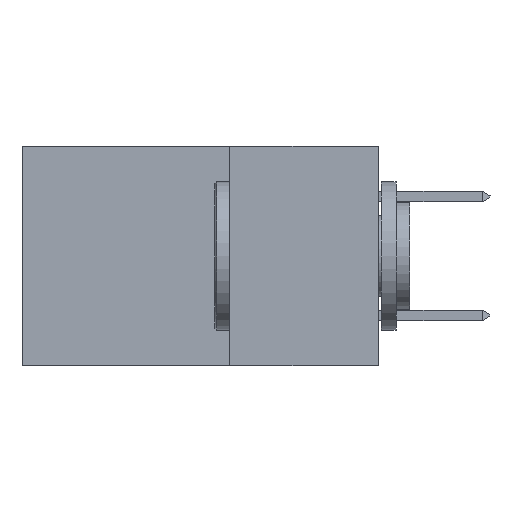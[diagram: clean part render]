
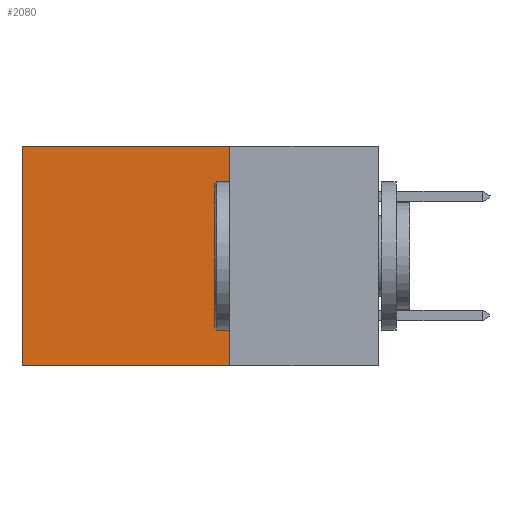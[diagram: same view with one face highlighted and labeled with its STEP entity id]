
A CAD part, left-side view. The second image highlights one B-rep face of the part: STEP entity #2080.
In plain terms, the highlighted planar face has unit normal (-1, 0, 0).
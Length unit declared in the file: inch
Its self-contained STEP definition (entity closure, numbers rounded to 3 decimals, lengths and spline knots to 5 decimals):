
#318 = DIRECTION ( 'NONE',  ( 1., 0., 0. ) ) ;
#596 = EDGE_CURVE ( 'NONE', #10384, #10099, #8486, .T. ) ;
#719 = CARTESIAN_POINT ( 'NONE',  ( 0.2615, 0.25, 0. ) ) ;
#1499 = CARTESIAN_POINT ( 'NONE',  ( 0.2615, 0.25, 0. ) ) ;
#1875 = CARTESIAN_POINT ( 'NONE',  ( 0.2615, 0.25, -0.37 ) ) ;
#2080 = ADVANCED_FACE ( 'NONE', ( #8927 ), #8737, .F. ) ;
#2107 = EDGE_LOOP ( 'NONE', ( #5415, #2706, #9807, #5911 ) ) ;
#2665 = VECTOR ( 'NONE', #9935, 39.37008 ) ;
#2706 = ORIENTED_EDGE ( 'NONE', *, *, #596, .F. ) ;
#3731 = CARTESIAN_POINT ( 'NONE',  ( 0.2615, 0.25, -0.37 ) ) ;
#4138 = AXIS2_PLACEMENT_3D ( 'NONE', #11734, #318, #5097 ) ;
#4532 = CARTESIAN_POINT ( 'NONE',  ( 0.2615, 0.6, -0.37 ) ) ;
#4996 = VERTEX_POINT ( 'NONE', #10766 ) ;
#5006 = CARTESIAN_POINT ( 'NONE',  ( 0.2615, 0.25, -0.37 ) ) ;
#5097 = DIRECTION ( 'NONE',  ( 0., 0., -1. ) ) ;
#5269 = VERTEX_POINT ( 'NONE', #719 ) ;
#5415 = ORIENTED_EDGE ( 'NONE', *, *, #12300, .T. ) ;
#5732 = VECTOR ( 'NONE', #9293, 39.37008 ) ;
#5911 = ORIENTED_EDGE ( 'NONE', *, *, #10007, .T. ) ;
#6651 = DIRECTION ( 'NONE',  ( 0., 1., 0. ) ) ;
#7490 = LINE ( 'NONE', #3731, #7873 ) ;
#7873 = VECTOR ( 'NONE', #12373, 39.37008 ) ;
#8486 = LINE ( 'NONE', #1875, #11488 ) ;
#8737 = PLANE ( 'NONE',  #4138 ) ;
#8927 = FACE_OUTER_BOUND ( 'NONE', #2107, .T. ) ;
#9163 = LINE ( 'NONE', #1499, #5732 ) ;
#9195 = LINE ( 'NONE', #10050, #2665 ) ;
#9293 = DIRECTION ( 'NONE',  ( 0., 1., 0. ) ) ;
#9807 = ORIENTED_EDGE ( 'NONE', *, *, #12343, .F. ) ;
#9935 = DIRECTION ( 'NONE',  ( 0., 0., -1. ) ) ;
#10007 = EDGE_CURVE ( 'NONE', #5269, #4996, #9163, .T. ) ;
#10050 = CARTESIAN_POINT ( 'NONE',  ( 0.2615, 0.6, -0.37 ) ) ;
#10099 = VERTEX_POINT ( 'NONE', #4532 ) ;
#10384 = VERTEX_POINT ( 'NONE', #5006 ) ;
#10766 = CARTESIAN_POINT ( 'NONE',  ( 0.2615, 0.6, 0. ) ) ;
#11488 = VECTOR ( 'NONE', #6651, 39.37008 ) ;
#11734 = CARTESIAN_POINT ( 'NONE',  ( 0.2615, 0.25, -0.37 ) ) ;
#12300 = EDGE_CURVE ( 'NONE', #4996, #10099, #9195, .T. ) ;
#12343 = EDGE_CURVE ( 'NONE', #5269, #10384, #7490, .T. ) ;
#12373 = DIRECTION ( 'NONE',  ( 0., 0., -1. ) ) ;
